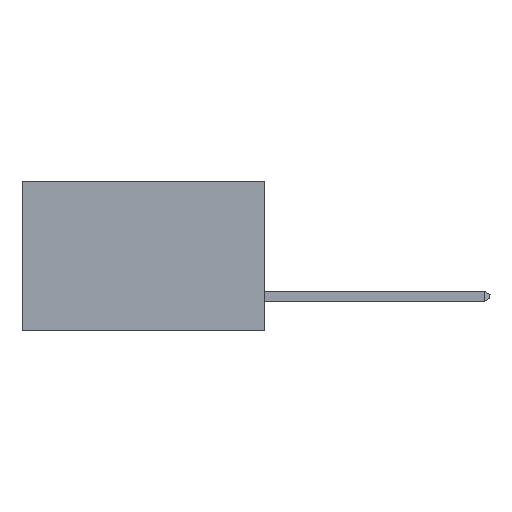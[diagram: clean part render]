
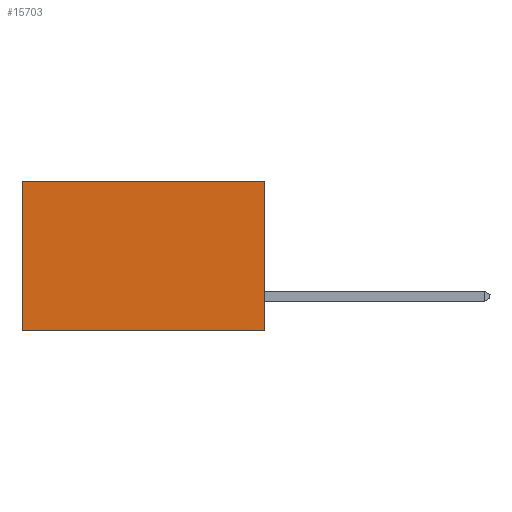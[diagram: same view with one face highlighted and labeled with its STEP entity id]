
A CAD part, left-side view. The second image highlights one B-rep face of the part: STEP entity #15703.
In plain terms, the highlighted planar face has unit normal (-1, 0, 0).
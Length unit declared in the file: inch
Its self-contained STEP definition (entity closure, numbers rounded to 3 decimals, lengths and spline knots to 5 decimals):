
#1570 = DIRECTION ( 'NONE',  ( 1., 0., 0. ) ) ;
#1653 = DIRECTION ( 'NONE',  ( 0., 1., 0. ) ) ;
#1858 = VERTEX_POINT ( 'NONE', #20120 ) ;
#3549 = LINE ( 'NONE', #17532, #13606 ) ;
#5094 = CARTESIAN_POINT ( 'NONE',  ( 0.298, 0., 0. ) ) ;
#7025 = VERTEX_POINT ( 'NONE', #5094 ) ;
#7982 = CARTESIAN_POINT ( 'NONE',  ( 0.298, 0., -0.37 ) ) ;
#9393 = CARTESIAN_POINT ( 'NONE',  ( 0.298, 0., 0. ) ) ;
#9416 = VERTEX_POINT ( 'NONE', #21045 ) ;
#9510 = EDGE_CURVE ( 'NONE', #24503, #1858, #3549, .T. ) ;
#9896 = DIRECTION ( 'NONE',  ( 0., 0., -1. ) ) ;
#9954 = DIRECTION ( 'NONE',  ( 0., 0., -1. ) ) ;
#9985 = DIRECTION ( 'NONE',  ( 0., 1., 0. ) ) ;
#10834 = LINE ( 'NONE', #21604, #29097 ) ;
#11186 = PLANE ( 'NONE',  #30709 ) ;
#11300 = CARTESIAN_POINT ( 'NONE',  ( 0.298, 0., 0. ) ) ;
#13606 = VECTOR ( 'NONE', #1653, 39.37008 ) ;
#15470 = ORIENTED_EDGE ( 'NONE', *, *, #9510, .F. ) ;
#15703 = ADVANCED_FACE ( 'NONE', ( #18123 ), #11186, .F. ) ;
#15758 = ORIENTED_EDGE ( 'NONE', *, *, #18063, .T. ) ;
#17532 = CARTESIAN_POINT ( 'NONE',  ( 0.298, 0., -0.37 ) ) ;
#18063 = EDGE_CURVE ( 'NONE', #7025, #9416, #28748, .T. ) ;
#18123 = FACE_OUTER_BOUND ( 'NONE', #18544, .T. ) ;
#18544 = EDGE_LOOP ( 'NONE', ( #22296, #15470, #22185, #15758 ) ) ;
#20120 = CARTESIAN_POINT ( 'NONE',  ( 0.298, 0.6, -0.37 ) ) ;
#21045 = CARTESIAN_POINT ( 'NONE',  ( 0.298, 0.6, 0. ) ) ;
#21604 = CARTESIAN_POINT ( 'NONE',  ( 0.298, 0., 0. ) ) ;
#22185 = ORIENTED_EDGE ( 'NONE', *, *, #24391, .F. ) ;
#22296 = ORIENTED_EDGE ( 'NONE', *, *, #28417, .T. ) ;
#24389 = CARTESIAN_POINT ( 'NONE',  ( 0.298, 0.6, 0. ) ) ;
#24391 = EDGE_CURVE ( 'NONE', #7025, #24503, #10834, .T. ) ;
#24503 = VERTEX_POINT ( 'NONE', #7982 ) ;
#24673 = LINE ( 'NONE', #24389, #29925 ) ;
#25568 = DIRECTION ( 'NONE',  ( 0., 0., -1. ) ) ;
#26133 = VECTOR ( 'NONE', #9985, 39.37008 ) ;
#28417 = EDGE_CURVE ( 'NONE', #9416, #1858, #24673, .T. ) ;
#28748 = LINE ( 'NONE', #9393, #26133 ) ;
#29097 = VECTOR ( 'NONE', #9954, 39.37008 ) ;
#29925 = VECTOR ( 'NONE', #9896, 39.37008 ) ;
#30709 = AXIS2_PLACEMENT_3D ( 'NONE', #11300, #1570, #25568 ) ;
